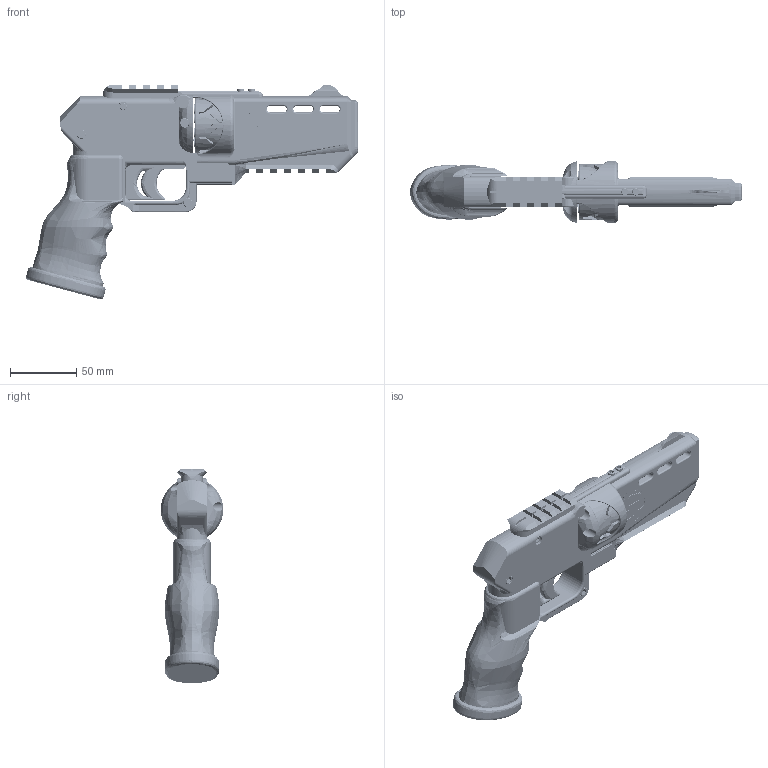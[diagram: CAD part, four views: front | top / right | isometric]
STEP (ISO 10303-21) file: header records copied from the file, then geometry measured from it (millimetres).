
FILE_DESCRIPTION(/* description */ (''),/* implementation_level */ '2;1');
FILE_NAME(/* name */ 'ImuraZip Final Working 22032020.step',/* time_stamp */ '2020-03-22T19:36:50+01:00',/* author */ (''),/* organization */ (''),/* preprocessor_version */ 'ST-DEVELOPER v18',/* originating_system */ 'Autodesk Translation Framework v8.12.0.6',/* authorisation */ '');
FILE_SCHEMA (('AUTOMOTIVE_DESIGN { 1 0 10303 214 3 1 1 }'));
Products named in the file (69): ImuraZip Final 17032020; ImuraZip; FrameParts; ImuraBarrel; Imura_V2_Cylinder; 22LR; Cylinder Rod 8mm; Cylinder; Chamber Inserts; Inserts 25mm x 5; Barrel Front; Locking Lever; Barrel; FramePin 23x5mm; Component53; Rail; RailPin; Rail (1); Frame; Half Right ; Right Frame; Cover Right; Release Pin 8mm; Component52; Half Left 1 Spring; Left Frame; Cover Left; Internals; ImuraTrigger; SpringTrigger 1 (1); SpringTrigger 2 (1); Trigger ; Trigger (1); ImuraSearV4; Sear; Pin (1); ImuraStriker; Firing Pin; Sriker; Spring (1) ...
Assembly tree (68 placements, depth 7):
  ImuraZip Final 17032020
    ImuraZip
      FrameParts
        ImuraBarrel
          Imura_V2_Cylinder
            22LR
            Cylinder Rod 8mm
            Cylinder
            Chamber Inserts
              Inserts 25mm x 5
          Barrel Front
          Locking Lever
          Barrel
          FramePin 23x5mm
            Component53
        Rail
          RailPin
          Rail (1)
        Frame
          Half Right 
            Right Frame
            Cover Right
          Release Pin 8mm
            Component52
          Half Left 1 Spring
            Left Frame
            Cover Left
        Internals
          ImuraTrigger
            SpringTrigger 1 (1)
            SpringTrigger 2 (1)
            Trigger 
              Trigger (1)
          ImuraSearV4
            Sear
            Pin (1)
          ImuraStriker
            Firing Pin
            Sriker
            Spring (1)
          ImuraFlapper
            FlapperSpring
            FlapperV4
            Pin
      Grip
        grip_1
        Bottom Plug
      Thread Inserts Not on Spec
        Threaded Insert M4 3
        Threaded Insert M4 2
        Threaded Insert M4
        Threaded Insert M3
        Threaded Insert M3 2
        Threaded Insert M3 3
        Threaded Insert M3 4
        Threaded Insert M3 5
      Screws
        M3 x 14mm
        M4 x 16mm
        M4 x 16mm 2
Bounding box: 250.11 x 47 x 161.71 mm (x, y, z)
Volume: 383263 mm3; surface area: 171774 mm2
Topology: 61 solids, 71 shells, 3667 faces, 10648 edges, 7314 vertices
Faces by surface type: bspline 1397, plane 1092, cylinder 891, cone 151, torus 104, sphere 32
Full cylindrical faces by diameter (mm): 0.793 x8, 1.5 x3, 2 x2, 2.356 x119, 2.459 x5, 3.053 x3, 3.25 x2, 3.3 x3, 3.5 x1, 3.6 x5, 4 x14, 4.1 x2, 4.2 x5, 4.25 x2, 4.469 x3, 4.5 x4, 4.7 x1, 4.8 x4, 4.965 x3, 5 x10, 5.1 x2, 5.3 x1, 5.4 x5, 5.5 x10, 5.56 x1, 5.588 x32, 5.6 x2, 5.69 x8, 5.715 x24, 6 x13
Entity records: 300919 total; most frequent: CARTESIAN_POINT 212634, ORIENTED_EDGE 21230, DIRECTION 13153, EDGE_CURVE 10615, VERTEX_POINT 7313, AXIS2_PLACEMENT_3D 4932, B_SPLINE_CURVE_WITH_KNOTS 4798, EDGE_LOOP 4012
